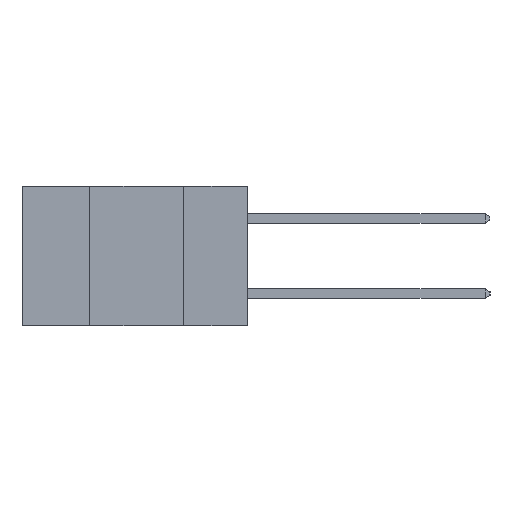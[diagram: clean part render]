
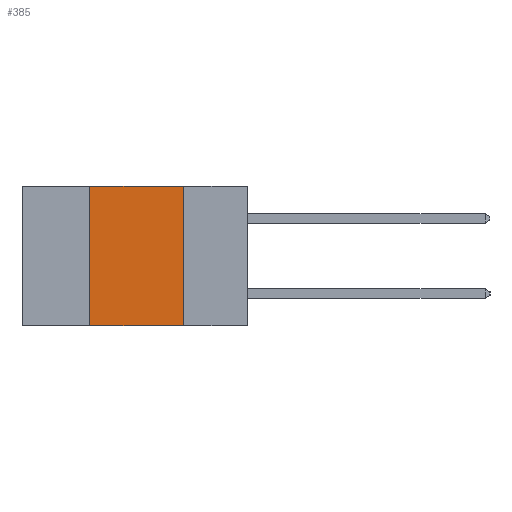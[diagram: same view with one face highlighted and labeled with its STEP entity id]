
A CAD part, left-side view. The second image highlights one B-rep face of the part: STEP entity #385.
In plain terms, the highlighted planar face has unit normal (-1, 0, 0).
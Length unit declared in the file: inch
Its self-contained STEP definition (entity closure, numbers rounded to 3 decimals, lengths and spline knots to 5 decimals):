
#385 = ADVANCED_FACE ( 'NONE', ( #817 ), #11623, .F. ) ;
#817 = FACE_OUTER_BOUND ( 'NONE', #1002, .T. ) ;
#1002 = EDGE_LOOP ( 'NONE', ( #7862, #3862, #14386, #1941 ) ) ;
#1583 = DIRECTION ( 'NONE',  ( 1., 0., 0. ) ) ;
#1922 = VECTOR ( 'NONE', #7145, 39.37008 ) ;
#1941 = ORIENTED_EDGE ( 'NONE', *, *, #6724, .T. ) ;
#2562 = VECTOR ( 'NONE', #4878, 39.37008 ) ;
#3750 = LINE ( 'NONE', #5073, #9404 ) ;
#3756 = VERTEX_POINT ( 'NONE', #11461 ) ;
#3760 = CARTESIAN_POINT ( 'NONE',  ( 0., 0.17, -0.37 ) ) ;
#3862 = ORIENTED_EDGE ( 'NONE', *, *, #10601, .F. ) ;
#3888 = VERTEX_POINT ( 'NONE', #10574 ) ;
#4878 = DIRECTION ( 'NONE',  ( 0., 0., -1. ) ) ;
#5016 = DIRECTION ( 'NONE',  ( 0., 0., 1. ) ) ;
#5073 = CARTESIAN_POINT ( 'NONE',  ( 0., 0.42, -0.37 ) ) ;
#5560 = DIRECTION ( 'NONE',  ( 0., 0., -1. ) ) ;
#5755 = CARTESIAN_POINT ( 'NONE',  ( 0., 0.6, 0. ) ) ;
#6724 = EDGE_CURVE ( 'NONE', #3756, #14317, #13807, .T. ) ;
#7145 = DIRECTION ( 'NONE',  ( 0., -1., 0. ) ) ;
#7373 = CARTESIAN_POINT ( 'NONE',  ( 0., 0.6, 0. ) ) ;
#7499 = EDGE_CURVE ( 'NONE', #3756, #12074, #3750, .T. ) ;
#7616 = CARTESIAN_POINT ( 'NONE',  ( 0., 0.17, -0.37 ) ) ;
#7862 = ORIENTED_EDGE ( 'NONE', *, *, #12851, .F. ) ;
#8516 = LINE ( 'NONE', #3760, #2562 ) ;
#9404 = VECTOR ( 'NONE', #5016, 39.37008 ) ;
#10377 = CARTESIAN_POINT ( 'NONE',  ( 0., 0.42, 0. ) ) ;
#10486 = VECTOR ( 'NONE', #10694, 39.37008 ) ;
#10574 = CARTESIAN_POINT ( 'NONE',  ( 0., 0.17, 0. ) ) ;
#10601 = EDGE_CURVE ( 'NONE', #12074, #3888, #10941, .T. ) ;
#10694 = DIRECTION ( 'NONE',  ( 0., -1., 0. ) ) ;
#10738 = CARTESIAN_POINT ( 'NONE',  ( 0., 0.6, -0.37 ) ) ;
#10941 = LINE ( 'NONE', #7373, #1922 ) ;
#11461 = CARTESIAN_POINT ( 'NONE',  ( 0., 0.42, -0.37 ) ) ;
#11623 = PLANE ( 'NONE',  #13391 ) ;
#12074 = VERTEX_POINT ( 'NONE', #10377 ) ;
#12851 = EDGE_CURVE ( 'NONE', #3888, #14317, #8516, .T. ) ;
#13391 = AXIS2_PLACEMENT_3D ( 'NONE', #5755, #1583, #5560 ) ;
#13807 = LINE ( 'NONE', #10738, #10486 ) ;
#14317 = VERTEX_POINT ( 'NONE', #7616 ) ;
#14386 = ORIENTED_EDGE ( 'NONE', *, *, #7499, .F. ) ;
